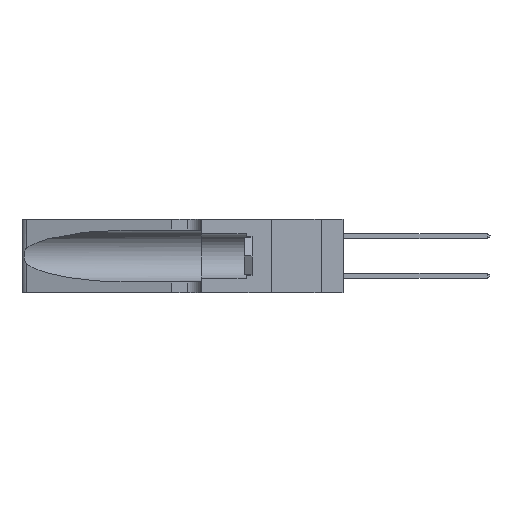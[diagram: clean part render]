
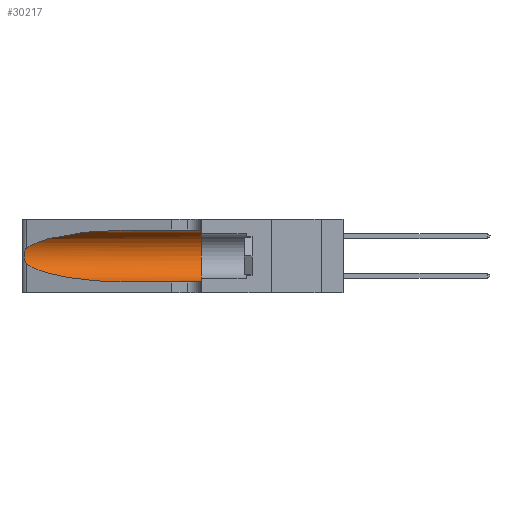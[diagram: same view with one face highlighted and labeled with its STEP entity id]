
A CAD part, left-side view. The second image highlights one B-rep face of the part: STEP entity #30217.
In plain terms, the highlighted cylindrical face has radius 3.308 mm (diameter 6.617 mm), a partial arc.
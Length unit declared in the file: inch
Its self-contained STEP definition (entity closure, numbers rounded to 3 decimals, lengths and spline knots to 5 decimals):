
#1797 = DIRECTION ( 'NONE',  ( 0., 0., 1. ) ) ;
#2548 = CARTESIAN_POINT ( 'NONE',  ( 0.25487, 1.22718, 0.22369 ) ) ;
#2809 = CARTESIAN_POINT ( 'NONE',  ( 0.25639, 1.23184, 0.21858 ) ) ;
#2894 = CARTESIAN_POINT ( 'NONE',  ( 0.25487, 1.22718, 0.22369 ) ) ;
#3452 = CARTESIAN_POINT ( 'NONE',  ( 0.18966, 0.96281, 0.05475 ) ) ;
#6103 = CARTESIAN_POINT ( 'NONE',  ( 0.25854, 1.2359, 0.20912 ) ) ;
#6644 = VERTEX_POINT ( 'NONE', #34273 ) ;
#7302 = AXIS2_PLACEMENT_3D ( 'NONE', #41495, #21995, #25310 ) ;
#8207 = CARTESIAN_POINT ( 'NONE',  ( 0.1305, 0.72297, 0.31525 ) ) ;
#9195 = VERTEX_POINT ( 'NONE', #8207 ) ;
#9412 = EDGE_CURVE ( 'NONE', #9195, #26238, #38529, .T. ) ;
#9421 = CARTESIAN_POINT ( 'NONE',  ( 0.26075, 1.23896, 0.19203 ) ) ;
#10315 = LINE ( 'NONE', #20475, #18070 ) ;
#11870 = AXIS2_PLACEMENT_3D ( 'NONE', #41019, #21514, #1797 ) ;
#12447 = VECTOR ( 'NONE', #35576, 39.37008 ) ;
#12606 = CARTESIAN_POINT ( 'NONE',  ( 0.25487, 1.22718, 0.22369 ) ) ;
#12741 = CARTESIAN_POINT ( 'NONE',  ( 0.26017, 1.23833, 0.17102 ) ) ;
#13163 = CARTESIAN_POINT ( 'NONE',  ( 0.25487, 1.22718, 0.14631 ) ) ;
#13293 = CIRCLE ( 'NONE', #11870, 0.13025 ) ;
#15619 = EDGE_CURVE ( 'NONE', #28935, #6644, #10315, .T. ) ;
#15687 = CARTESIAN_POINT ( 'NONE',  ( 0.1305, 0.72297, 0.31525 ) ) ;
#16073 = CARTESIAN_POINT ( 'NONE',  ( 0.25789, 1.23486, 0.15765 ) ) ;
#17656 = EDGE_LOOP ( 'NONE', ( #42183, #36630, #22341, #32080, #18187, #35568 ) ) ;
#17954 = EDGE_CURVE ( 'NONE', #26238, #6644, #13293, .T. ) ;
#18070 = VECTOR ( 'NONE', #39975, 39.37008 ) ;
#18187 = ORIENTED_EDGE ( 'NONE', *, *, #17954, .F. ) ;
#18990 = CARTESIAN_POINT ( 'NONE',  ( 0.18966, 0.96281, 0.31525 ) ) ;
#19386 = CARTESIAN_POINT ( 'NONE',  ( 0.25555, 1.22993, 0.14849 ) ) ;
#20475 = CARTESIAN_POINT ( 'NONE',  ( 0.1305, 1.61858, 0.05475 ) ) ;
#20535 = CYLINDRICAL_SURFACE ( 'NONE', #7302, 0.13025 ) ;
#21514 = DIRECTION ( 'NONE',  ( 0., 1., 0. ) ) ;
#21564 = FACE_OUTER_BOUND ( 'NONE', #17656, .T. ) ;
#21995 = DIRECTION ( 'NONE',  ( 0., -1., 0. ) ) ;
#22280 = CARTESIAN_POINT ( 'NONE',  ( 0.2373, 1.15595, 0.28018 ) ) ;
#22341 = ORIENTED_EDGE ( 'NONE', *, *, #36103, .T. ) ;
#22357 = CARTESIAN_POINT ( 'NONE',  ( 0.2373, 1.15595, 0.08982 ) ) ;
#22666 =( BOUNDED_CURVE ( )  B_SPLINE_CURVE ( 3, ( #15687, #18990, #22280, #2548 ),
 .UNSPECIFIED., .F., .T. ) 
 B_SPLINE_CURVE_WITH_KNOTS ( ( 4, 4 ),
 ( 1.5708, 2.84003 ),
 .UNSPECIFIED. ) 
 CURVE ( )  GEOMETRIC_REPRESENTATION_ITEM ( )  RATIONAL_B_SPLINE_CURVE ( ( 1., 0.87, 0.87, 1. ) ) 
 REPRESENTATION_ITEM ( '' )  );
#25075 = VERTEX_POINT ( 'NONE', #13163 ) ;
#25310 = DIRECTION ( 'NONE',  ( 0., 0., -1. ) ) ;
#25844 = CARTESIAN_POINT ( 'NONE',  ( 0.25787, 1.23484, 0.2124 ) ) ;
#26238 = VERTEX_POINT ( 'NONE', #40798 ) ;
#26475 = CARTESIAN_POINT ( 'NONE',  ( 0.1305, 0.72297, 0.05475 ) ) ;
#27180 = B_SPLINE_CURVE_WITH_KNOTS ( 'NONE', 3,
 ( #12606, #32265, #2809, #25844, #6103, #29160, #9421, #32403, #12741, #35673, #16073, #38886, #19386, #42162 ),
 .UNSPECIFIED., .F., .F.,
 ( 4, 2, 2, 2, 2, 2, 4 ),
 ( 0., 0.00027, 0.00053, 0.00107, 0.0016, 0.00187, 0.00214 ),
 .UNSPECIFIED. ) ;
#28422 = EDGE_CURVE ( 'NONE', #9195, #40372, #22666, .T. ) ;
#28935 = VERTEX_POINT ( 'NONE', #34535 ) ;
#29068 = CARTESIAN_POINT ( 'NONE',  ( 0.1305, 1.61858, 0.31525 ) ) ;
#29160 = CARTESIAN_POINT ( 'NONE',  ( 0.26018, 1.23835, 0.19895 ) ) ;
#30217 = ADVANCED_FACE ( 'NONE', ( #21564 ), #20535, .F. ) ;
#32080 = ORIENTED_EDGE ( 'NONE', *, *, #15619, .T. ) ;
#32265 = CARTESIAN_POINT ( 'NONE',  ( 0.25555, 1.22994, 0.2215 ) ) ;
#32403 = CARTESIAN_POINT ( 'NONE',  ( 0.26075, 1.23896, 0.178 ) ) ;
#34273 = CARTESIAN_POINT ( 'NONE',  ( 0.1305, 0.35, 0.05475 ) ) ;
#34535 = CARTESIAN_POINT ( 'NONE',  ( 0.1305, 0.72297, 0.05475 ) ) ;
#34731 =( BOUNDED_CURVE ( )  B_SPLINE_CURVE ( 3, ( #39367, #22357, #3452, #26475 ),
 .UNSPECIFIED., .F., .F. ) 
 B_SPLINE_CURVE_WITH_KNOTS ( ( 4, 4 ),
 ( 3.44316, 4.71239 ),
 .UNSPECIFIED. ) 
 CURVE ( )  GEOMETRIC_REPRESENTATION_ITEM ( )  RATIONAL_B_SPLINE_CURVE ( ( 1., 0.87, 0.87, 1. ) ) 
 REPRESENTATION_ITEM ( '' )  );
#35568 = ORIENTED_EDGE ( 'NONE', *, *, #9412, .F. ) ;
#35576 = DIRECTION ( 'NONE',  ( 0., -1., 0. ) ) ;
#35673 = CARTESIAN_POINT ( 'NONE',  ( 0.25856, 1.23593, 0.16098 ) ) ;
#36103 = EDGE_CURVE ( 'NONE', #25075, #28935, #34731, .T. ) ;
#36599 = EDGE_CURVE ( 'NONE', #40372, #25075, #27180, .T. ) ;
#36630 = ORIENTED_EDGE ( 'NONE', *, *, #36599, .T. ) ;
#38529 = LINE ( 'NONE', #29068, #12447 ) ;
#38886 = CARTESIAN_POINT ( 'NONE',  ( 0.25639, 1.23186, 0.15144 ) ) ;
#39367 = CARTESIAN_POINT ( 'NONE',  ( 0.25487, 1.22718, 0.14631 ) ) ;
#39975 = DIRECTION ( 'NONE',  ( 0., -1., 0. ) ) ;
#40372 = VERTEX_POINT ( 'NONE', #2894 ) ;
#40798 = CARTESIAN_POINT ( 'NONE',  ( 0.1305, 0.35, 0.31525 ) ) ;
#41019 = CARTESIAN_POINT ( 'NONE',  ( 0.1305, 0.35, 0.185 ) ) ;
#41495 = CARTESIAN_POINT ( 'NONE',  ( 0.1305, 1.61858, 0.185 ) ) ;
#42162 = CARTESIAN_POINT ( 'NONE',  ( 0.25487, 1.22718, 0.14631 ) ) ;
#42183 = ORIENTED_EDGE ( 'NONE', *, *, #28422, .T. ) ;
